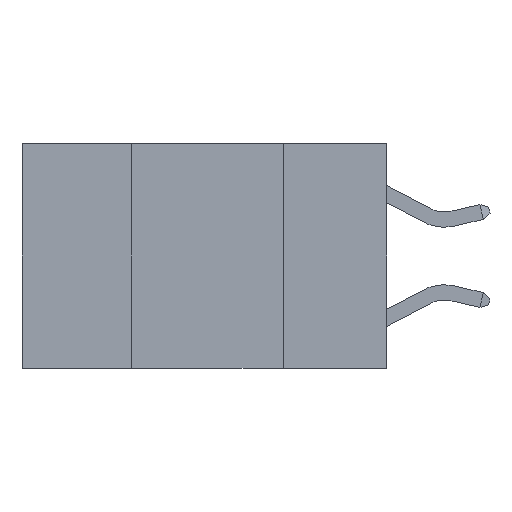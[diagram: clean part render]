
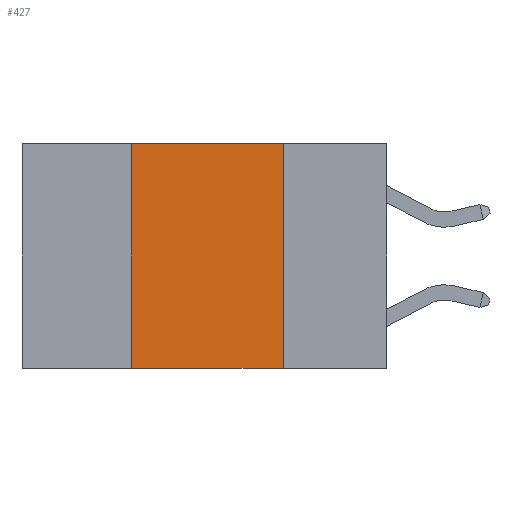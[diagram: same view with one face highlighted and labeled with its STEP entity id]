
A CAD part, left-side view. The second image highlights one B-rep face of the part: STEP entity #427.
In plain terms, the highlighted planar face has unit normal (-1, 0, 0).
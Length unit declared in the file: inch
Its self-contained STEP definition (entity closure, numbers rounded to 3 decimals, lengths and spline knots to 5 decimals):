
#75 = CARTESIAN_POINT ( 'NONE',  ( 0., 0.17, 0. ) ) ;
#215 = ORIENTED_EDGE ( 'NONE', *, *, #8436, .F. ) ;
#369 = DIRECTION ( 'NONE',  ( 0., 0., -1. ) ) ;
#427 = ADVANCED_FACE ( 'NONE', ( #7678 ), #7535, .F. ) ;
#450 = CARTESIAN_POINT ( 'NONE',  ( 0., 0.6, 0. ) ) ;
#703 = VERTEX_POINT ( 'NONE', #4476 ) ;
#861 = VECTOR ( 'NONE', #4182, 39.37008 ) ;
#1343 = LINE ( 'NONE', #2226, #861 ) ;
#1430 = DIRECTION ( 'NONE',  ( 0., 0., -1. ) ) ;
#1731 = LINE ( 'NONE', #75, #6549 ) ;
#2226 = CARTESIAN_POINT ( 'NONE',  ( 0., 0.42, 0. ) ) ;
#2260 = DIRECTION ( 'NONE',  ( 0., -1., 0. ) ) ;
#2594 = CARTESIAN_POINT ( 'NONE',  ( 0., 0.42, 0. ) ) ;
#2694 = EDGE_CURVE ( 'NONE', #7827, #703, #1731, .T. ) ;
#3382 = VECTOR ( 'NONE', #7291, 39.37008 ) ;
#4180 = ORIENTED_EDGE ( 'NONE', *, *, #2694, .F. ) ;
#4182 = DIRECTION ( 'NONE',  ( 0., 0., 1. ) ) ;
#4235 = EDGE_CURVE ( 'NONE', #8051, #703, #5076, .T. ) ;
#4476 = CARTESIAN_POINT ( 'NONE',  ( 0., 0.17, -0.37 ) ) ;
#4601 = VECTOR ( 'NONE', #2260, 39.37008 ) ;
#4957 = CARTESIAN_POINT ( 'NONE',  ( 0., 0.17, 0. ) ) ;
#5076 = LINE ( 'NONE', #7313, #3382 ) ;
#5189 = CARTESIAN_POINT ( 'NONE',  ( 0., 0.42, -0.37 ) ) ;
#5470 = LINE ( 'NONE', #6152, #4601 ) ;
#5828 = AXIS2_PLACEMENT_3D ( 'NONE', #450, #6164, #1430 ) ;
#5904 = EDGE_CURVE ( 'NONE', #8019, #7827, #5470, .T. ) ;
#6152 = CARTESIAN_POINT ( 'NONE',  ( 0., 0.6, 0. ) ) ;
#6164 = DIRECTION ( 'NONE',  ( 1., 0., 0. ) ) ;
#6190 = EDGE_LOOP ( 'NONE', ( #4180, #7748, #215, #6381 ) ) ;
#6381 = ORIENTED_EDGE ( 'NONE', *, *, #4235, .T. ) ;
#6549 = VECTOR ( 'NONE', #369, 39.37008 ) ;
#7291 = DIRECTION ( 'NONE',  ( 0., -1., 0. ) ) ;
#7313 = CARTESIAN_POINT ( 'NONE',  ( 0., 0.6, -0.37 ) ) ;
#7535 = PLANE ( 'NONE',  #5828 ) ;
#7678 = FACE_OUTER_BOUND ( 'NONE', #6190, .T. ) ;
#7748 = ORIENTED_EDGE ( 'NONE', *, *, #5904, .F. ) ;
#7827 = VERTEX_POINT ( 'NONE', #4957 ) ;
#8019 = VERTEX_POINT ( 'NONE', #2594 ) ;
#8051 = VERTEX_POINT ( 'NONE', #5189 ) ;
#8436 = EDGE_CURVE ( 'NONE', #8051, #8019, #1343, .T. ) ;
